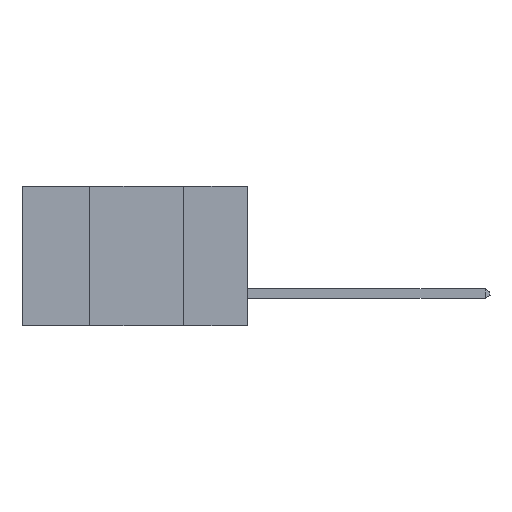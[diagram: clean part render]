
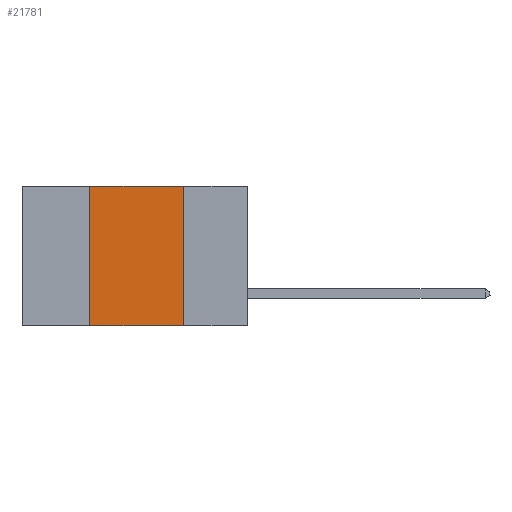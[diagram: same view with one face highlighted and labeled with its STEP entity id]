
A CAD part, left-side view. The second image highlights one B-rep face of the part: STEP entity #21781.
In plain terms, the highlighted planar face has unit normal (-1, 0, 0).
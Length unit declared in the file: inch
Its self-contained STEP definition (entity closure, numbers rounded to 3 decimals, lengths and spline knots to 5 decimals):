
#226 = CARTESIAN_POINT ( 'NONE',  ( 0., 0.17, 0. ) ) ;
#1417 = PLANE ( 'NONE',  #4604 ) ;
#1938 = CARTESIAN_POINT ( 'NONE',  ( 0., 0.42, 0. ) ) ;
#2147 = LINE ( 'NONE', #8727, #14156 ) ;
#2262 = VERTEX_POINT ( 'NONE', #1938 ) ;
#2405 = VECTOR ( 'NONE', #5199, 39.37008 ) ;
#2524 = CARTESIAN_POINT ( 'NONE',  ( 0., 0.42, -0.37 ) ) ;
#3505 = CARTESIAN_POINT ( 'NONE',  ( 0., 0.6, 0. ) ) ;
#4604 = AXIS2_PLACEMENT_3D ( 'NONE', #13031, #21730, #11398 ) ;
#4671 = ORIENTED_EDGE ( 'NONE', *, *, #21422, .F. ) ;
#5199 = DIRECTION ( 'NONE',  ( 0., -1., 0. ) ) ;
#5564 = VERTEX_POINT ( 'NONE', #2524 ) ;
#6800 = DIRECTION ( 'NONE',  ( 0., 0., -1. ) ) ;
#7293 = ORIENTED_EDGE ( 'NONE', *, *, #14693, .F. ) ;
#8727 = CARTESIAN_POINT ( 'NONE',  ( 0., 0.42, 0. ) ) ;
#10642 = ORIENTED_EDGE ( 'NONE', *, *, #21449, .F. ) ;
#10652 = VECTOR ( 'NONE', #6800, 39.37008 ) ;
#10937 = DIRECTION ( 'NONE',  ( 0., -1., 0. ) ) ;
#11177 = LINE ( 'NONE', #16738, #10652 ) ;
#11398 = DIRECTION ( 'NONE',  ( 0., 0., -1. ) ) ;
#11629 = EDGE_LOOP ( 'NONE', ( #7293, #4671, #10642, #20594 ) ) ;
#13031 = CARTESIAN_POINT ( 'NONE',  ( 0., 0.6, 0. ) ) ;
#13812 = VERTEX_POINT ( 'NONE', #226 ) ;
#13838 = VERTEX_POINT ( 'NONE', #20446 ) ;
#14156 = VECTOR ( 'NONE', #20751, 39.37008 ) ;
#14693 = EDGE_CURVE ( 'NONE', #13812, #13838, #11177, .T. ) ;
#16201 = EDGE_CURVE ( 'NONE', #5564, #13838, #17116, .T. ) ;
#16738 = CARTESIAN_POINT ( 'NONE',  ( 0., 0.17, 0. ) ) ;
#17116 = LINE ( 'NONE', #19236, #19797 ) ;
#17314 = FACE_OUTER_BOUND ( 'NONE', #11629, .T. ) ;
#19236 = CARTESIAN_POINT ( 'NONE',  ( 0., 0.6, -0.37 ) ) ;
#19797 = VECTOR ( 'NONE', #10937, 39.37008 ) ;
#20446 = CARTESIAN_POINT ( 'NONE',  ( 0., 0.17, -0.37 ) ) ;
#20569 = LINE ( 'NONE', #3505, #2405 ) ;
#20594 = ORIENTED_EDGE ( 'NONE', *, *, #16201, .T. ) ;
#20751 = DIRECTION ( 'NONE',  ( 0., 0., 1. ) ) ;
#21422 = EDGE_CURVE ( 'NONE', #2262, #13812, #20569, .T. ) ;
#21449 = EDGE_CURVE ( 'NONE', #5564, #2262, #2147, .T. ) ;
#21730 = DIRECTION ( 'NONE',  ( 1., 0., 0. ) ) ;
#21781 = ADVANCED_FACE ( 'NONE', ( #17314 ), #1417, .F. ) ;
